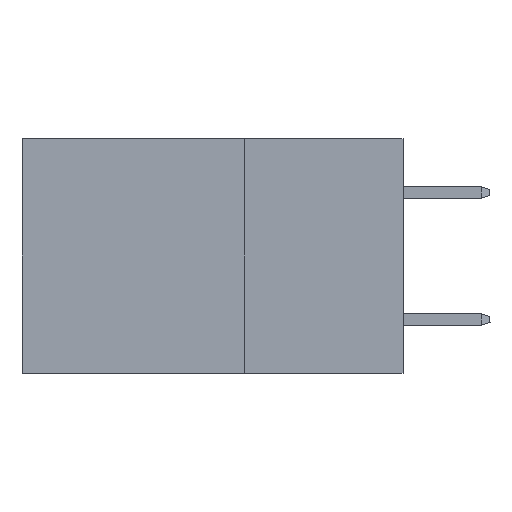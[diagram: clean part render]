
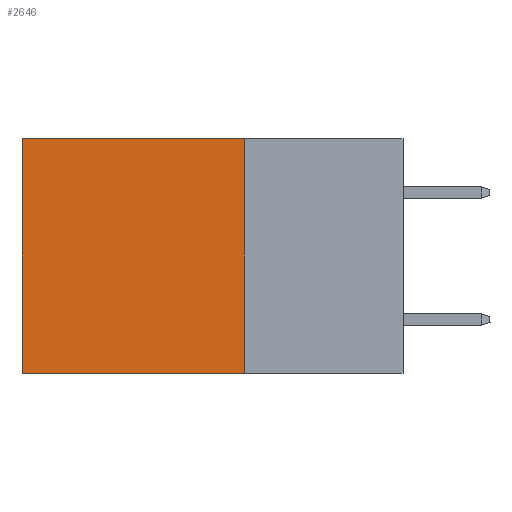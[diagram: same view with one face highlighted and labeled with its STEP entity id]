
A CAD part, left-side view. The second image highlights one B-rep face of the part: STEP entity #2646.
In plain terms, the highlighted planar face has unit normal (-1, 0, 0).
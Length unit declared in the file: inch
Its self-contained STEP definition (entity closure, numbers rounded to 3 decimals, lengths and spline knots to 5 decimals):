
#498 = EDGE_CURVE ( 'NONE', #12055, #705, #12576, .T. ) ;
#705 = VERTEX_POINT ( 'NONE', #5016 ) ;
#710 = ORIENTED_EDGE ( 'NONE', *, *, #2735, .T. ) ;
#1027 = ORIENTED_EDGE ( 'NONE', *, *, #498, .T. ) ;
#1339 = LINE ( 'NONE', #8368, #6940 ) ;
#1730 = VERTEX_POINT ( 'NONE', #4394 ) ;
#2646 = ADVANCED_FACE ( 'NONE', ( #13269 ), #3507, .F. ) ;
#2735 = EDGE_CURVE ( 'NONE', #13748, #12055, #16244, .T. ) ;
#3421 = CARTESIAN_POINT ( 'NONE',  ( 0.2875, 0.25, 0. ) ) ;
#3507 = PLANE ( 'NONE',  #12643 ) ;
#4108 = DIRECTION ( 'NONE',  ( 0., 1., 0. ) ) ;
#4394 = CARTESIAN_POINT ( 'NONE',  ( 0.2875, 0.25, -0.37 ) ) ;
#4652 = DIRECTION ( 'NONE',  ( 0., 0., -1. ) ) ;
#4746 = CARTESIAN_POINT ( 'NONE',  ( 0.2875, 0.25, 0. ) ) ;
#5016 = CARTESIAN_POINT ( 'NONE',  ( 0.2875, 0.6, -0.37 ) ) ;
#5312 = VECTOR ( 'NONE', #10454, 39.37008 ) ;
#5597 = ORIENTED_EDGE ( 'NONE', *, *, #11754, .F. ) ;
#5865 = CARTESIAN_POINT ( 'NONE',  ( 0.2875, 0.6, 0. ) ) ;
#6197 = ORIENTED_EDGE ( 'NONE', *, *, #12071, .F. ) ;
#6220 = CARTESIAN_POINT ( 'NONE',  ( 0.2875, 0.6, 0. ) ) ;
#6940 = VECTOR ( 'NONE', #4108, 39.37008 ) ;
#7533 = CARTESIAN_POINT ( 'NONE',  ( 0.2875, 0.25, 0. ) ) ;
#8368 = CARTESIAN_POINT ( 'NONE',  ( 0.2875, 0.25, -0.37 ) ) ;
#8516 = CARTESIAN_POINT ( 'NONE',  ( 0.2875, 0.25, 0. ) ) ;
#8670 = VECTOR ( 'NONE', #4652, 39.37008 ) ;
#10370 = DIRECTION ( 'NONE',  ( 0., 0., -1. ) ) ;
#10454 = DIRECTION ( 'NONE',  ( 0., 1., 0. ) ) ;
#11754 = EDGE_CURVE ( 'NONE', #1730, #705, #1339, .T. ) ;
#12055 = VERTEX_POINT ( 'NONE', #6220 ) ;
#12071 = EDGE_CURVE ( 'NONE', #13748, #1730, #17172, .T. ) ;
#12576 = LINE ( 'NONE', #5865, #17803 ) ;
#12643 = AXIS2_PLACEMENT_3D ( 'NONE', #4746, #17348, #10370 ) ;
#13104 = DIRECTION ( 'NONE',  ( 0., 0., -1. ) ) ;
#13269 = FACE_OUTER_BOUND ( 'NONE', #17774, .T. ) ;
#13748 = VERTEX_POINT ( 'NONE', #8516 ) ;
#16244 = LINE ( 'NONE', #7533, #5312 ) ;
#17172 = LINE ( 'NONE', #3421, #8670 ) ;
#17348 = DIRECTION ( 'NONE',  ( 1., 0., 0. ) ) ;
#17774 = EDGE_LOOP ( 'NONE', ( #1027, #5597, #6197, #710 ) ) ;
#17803 = VECTOR ( 'NONE', #13104, 39.37008 ) ;
